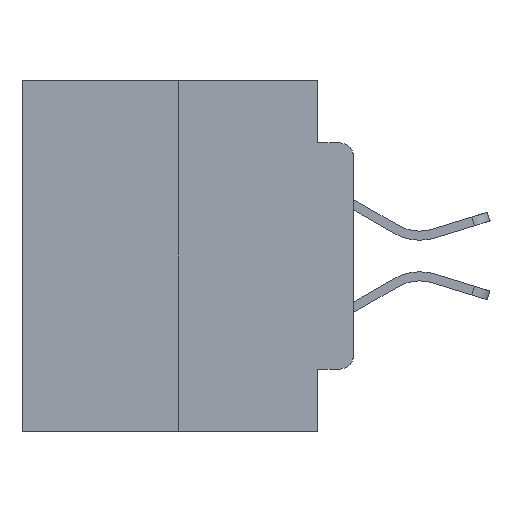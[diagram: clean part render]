
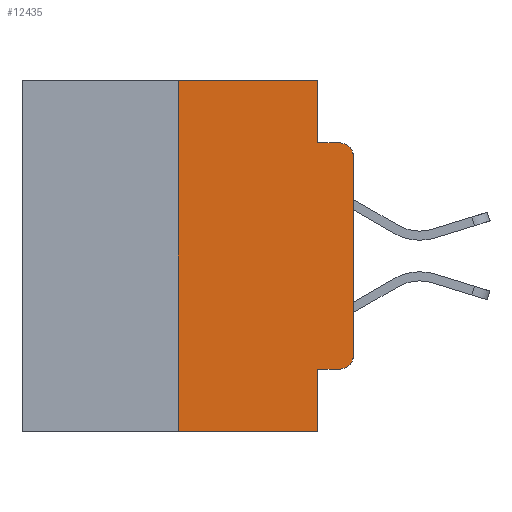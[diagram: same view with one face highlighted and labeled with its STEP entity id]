
A CAD part, left-side view. The second image highlights one B-rep face of the part: STEP entity #12435.
In plain terms, the highlighted planar face has unit normal (-1, 0, 0).
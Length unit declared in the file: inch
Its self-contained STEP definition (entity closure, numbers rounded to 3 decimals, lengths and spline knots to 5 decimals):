
#242 = VERTEX_POINT ( 'NONE', #15566 ) ;
#612 = EDGE_CURVE ( 'NONE', #17429, #7154, #1081, .T. ) ;
#900 = CARTESIAN_POINT ( 'NONE',  ( 0., 0., -0.3915 ) ) ;
#1081 = CIRCLE ( 'NONE', #21770, 0.02 ) ;
#1314 = CARTESIAN_POINT ( 'NONE',  ( 0., 0.25, 0. ) ) ;
#3157 = ORIENTED_EDGE ( 'NONE', *, *, #12474, .T. ) ;
#3339 = CARTESIAN_POINT ( 'NONE',  ( 0., 0.051, 0. ) ) ;
#3585 = PLANE ( 'NONE',  #13079 ) ;
#3614 = EDGE_CURVE ( 'NONE', #8594, #17429, #16034, .T. ) ;
#3894 = VERTEX_POINT ( 'NONE', #14010 ) ;
#5116 = EDGE_CURVE ( 'NONE', #8594, #3894, #19624, .T. ) ;
#5296 = VERTEX_POINT ( 'NONE', #22705 ) ;
#5451 = LINE ( 'NONE', #14388, #11996 ) ;
#6297 = VECTOR ( 'NONE', #16590, 39.37008 ) ;
#6501 = CARTESIAN_POINT ( 'NONE',  ( 0., 0.473, -0.5 ) ) ;
#6591 = EDGE_CURVE ( 'NONE', #14555, #5296, #18452, .T. ) ;
#6861 = VECTOR ( 'NONE', #19557, 39.37008 ) ;
#7154 = VERTEX_POINT ( 'NONE', #900 ) ;
#7327 = DIRECTION ( 'NONE',  ( -1., 0., 0. ) ) ;
#8029 = DIRECTION ( 'NONE',  ( 0., 0., -1. ) ) ;
#8064 = EDGE_CURVE ( 'NONE', #23940, #242, #26663, .T. ) ;
#8594 = VERTEX_POINT ( 'NONE', #27032 ) ;
#8637 = LINE ( 'NONE', #27294, #20063 ) ;
#8727 = DIRECTION ( 'NONE',  ( 0., -1., 0. ) ) ;
#9279 = LINE ( 'NONE', #6501, #19340 ) ;
#9539 = EDGE_CURVE ( 'NONE', #242, #11589, #12694, .T. ) ;
#9698 = VECTOR ( 'NONE', #10554, 39.37008 ) ;
#10554 = DIRECTION ( 'NONE',  ( 0., 0., -1. ) ) ;
#10561 = CIRCLE ( 'NONE', #18547, 0.02 ) ;
#11005 = EDGE_CURVE ( 'NONE', #17990, #11589, #10561, .T. ) ;
#11310 = ORIENTED_EDGE ( 'NONE', *, *, #24722, .T. ) ;
#11451 = DIRECTION ( 'NONE',  ( 0., 0., -1. ) ) ;
#11589 = VERTEX_POINT ( 'NONE', #15557 ) ;
#11996 = VECTOR ( 'NONE', #22839, 39.37008 ) ;
#12435 = ADVANCED_FACE ( 'NONE', ( #20702 ), #3585, .F. ) ;
#12474 = EDGE_CURVE ( 'NONE', #7154, #17990, #8637, .T. ) ;
#12694 = LINE ( 'NONE', #27898, #6861 ) ;
#13079 = AXIS2_PLACEMENT_3D ( 'NONE', #18733, #20884, #8029 ) ;
#13131 = ORIENTED_EDGE ( 'NONE', *, *, #612, .T. ) ;
#14010 = CARTESIAN_POINT ( 'NONE',  ( 0., 0.051, -0.5 ) ) ;
#14388 = CARTESIAN_POINT ( 'NONE',  ( 0., 0.473, 0. ) ) ;
#14555 = VERTEX_POINT ( 'NONE', #18484 ) ;
#14656 = DIRECTION ( 'NONE',  ( 0., 0., 1. ) ) ;
#15099 = CARTESIAN_POINT ( 'NONE',  ( 0., 0.02, -0.4115 ) ) ;
#15557 = CARTESIAN_POINT ( 'NONE',  ( 0., 0.02, -0.0885 ) ) ;
#15566 = CARTESIAN_POINT ( 'NONE',  ( 0., 0.051, -0.0885 ) ) ;
#15674 = CARTESIAN_POINT ( 'NONE',  ( 0., 0.051, 0. ) ) ;
#16034 = LINE ( 'NONE', #20595, #20363 ) ;
#16170 = ORIENTED_EDGE ( 'NONE', *, *, #3614, .T. ) ;
#16326 = ORIENTED_EDGE ( 'NONE', *, *, #6591, .F. ) ;
#16590 = DIRECTION ( 'NONE',  ( 0., 0., 1. ) ) ;
#16840 = ORIENTED_EDGE ( 'NONE', *, *, #25085, .F. ) ;
#16894 = CARTESIAN_POINT ( 'NONE',  ( 0., 0.051, 0. ) ) ;
#17350 = ORIENTED_EDGE ( 'NONE', *, *, #5116, .F. ) ;
#17429 = VERTEX_POINT ( 'NONE', #15099 ) ;
#17667 = ORIENTED_EDGE ( 'NONE', *, *, #9539, .F. ) ;
#17990 = VERTEX_POINT ( 'NONE', #27330 ) ;
#18452 = LINE ( 'NONE', #1314, #6297 ) ;
#18484 = CARTESIAN_POINT ( 'NONE',  ( 0., 0.25, -0.5 ) ) ;
#18547 = AXIS2_PLACEMENT_3D ( 'NONE', #20224, #7327, #22334 ) ;
#18680 = EDGE_LOOP ( 'NONE', ( #3157, #21406, #17667, #23792, #16840, #16326, #11310, #17350, #16170, #13131 ) ) ;
#18733 = CARTESIAN_POINT ( 'NONE',  ( 0., 0.473, 0. ) ) ;
#19340 = VECTOR ( 'NONE', #8727, 39.37008 ) ;
#19557 = DIRECTION ( 'NONE',  ( 0., -1., 0. ) ) ;
#19624 = LINE ( 'NONE', #15674, #24570 ) ;
#20063 = VECTOR ( 'NONE', #14656, 39.37008 ) ;
#20224 = CARTESIAN_POINT ( 'NONE',  ( 0., 0.02, -0.1085 ) ) ;
#20363 = VECTOR ( 'NONE', #20587, 39.37008 ) ;
#20587 = DIRECTION ( 'NONE',  ( 0., -1., 0. ) ) ;
#20595 = CARTESIAN_POINT ( 'NONE',  ( 0., 0.051, -0.4115 ) ) ;
#20702 = FACE_OUTER_BOUND ( 'NONE', #18680, .T. ) ;
#20884 = DIRECTION ( 'NONE',  ( 1., 0., 0. ) ) ;
#21406 = ORIENTED_EDGE ( 'NONE', *, *, #11005, .T. ) ;
#21770 = AXIS2_PLACEMENT_3D ( 'NONE', #23007, #22920, #22828 ) ;
#22334 = DIRECTION ( 'NONE',  ( 0., 0., -1. ) ) ;
#22705 = CARTESIAN_POINT ( 'NONE',  ( 0., 0.25, 0. ) ) ;
#22828 = DIRECTION ( 'NONE',  ( 0., 0., -1. ) ) ;
#22839 = DIRECTION ( 'NONE',  ( 0., -1., 0. ) ) ;
#22920 = DIRECTION ( 'NONE',  ( -1., 0., 0. ) ) ;
#23007 = CARTESIAN_POINT ( 'NONE',  ( 0., 0.02, -0.3915 ) ) ;
#23792 = ORIENTED_EDGE ( 'NONE', *, *, #8064, .F. ) ;
#23940 = VERTEX_POINT ( 'NONE', #3339 ) ;
#24570 = VECTOR ( 'NONE', #11451, 39.37008 ) ;
#24722 = EDGE_CURVE ( 'NONE', #14555, #3894, #9279, .T. ) ;
#25085 = EDGE_CURVE ( 'NONE', #5296, #23940, #5451, .T. ) ;
#26663 = LINE ( 'NONE', #16894, #9698 ) ;
#27032 = CARTESIAN_POINT ( 'NONE',  ( 0., 0.051, -0.4115 ) ) ;
#27294 = CARTESIAN_POINT ( 'NONE',  ( 0., 0., 0. ) ) ;
#27330 = CARTESIAN_POINT ( 'NONE',  ( 0., 0., -0.1085 ) ) ;
#27898 = CARTESIAN_POINT ( 'NONE',  ( 0., 0.051, -0.0885 ) ) ;
